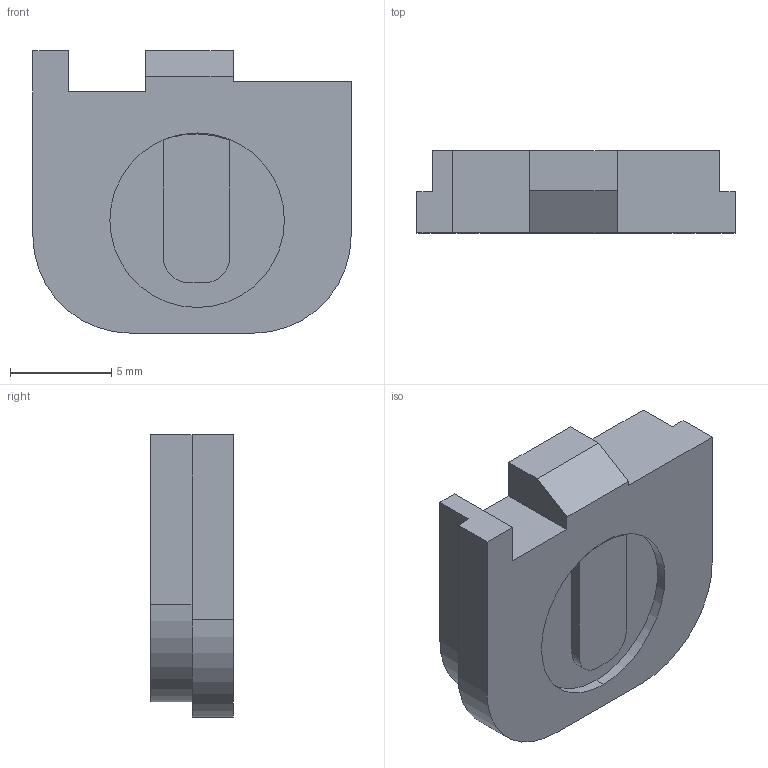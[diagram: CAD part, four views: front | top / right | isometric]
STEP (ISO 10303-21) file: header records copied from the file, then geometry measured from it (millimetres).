
FILE_DESCRIPTION (( 'STEP AP203' ), '1' );
FILE_NAME ('48BPv3.STEP', '2020-08-02T20:02:58', ( '' ), ( '' ), 'SwSTEP 2.0', 'SolidWorks 2020', '' );
FILE_SCHEMA (( 'CONFIG_CONTROL_DESIGN' ));
Length unit declared in the file: inch
Products named in the file (1): 48BPv3
Bounding box: 15.75 x 4.06 x 13.97 mm (x, y, z)
Volume: 699.2 mm3; surface area: 682.4 mm2
Topology: 2 solids, 2 shells, 32 faces, 81 edges, 54 vertices
Faces by surface type: plane 23, cylinder 8, bspline 1
Entity records: 1040 total; most frequent: CARTESIAN_POINT 177, ORIENTED_EDGE 162, DIRECTION 159, EDGE_CURVE 81, VECTOR 63, LINE 63, VERTEX_POINT 54, AXIS2_PLACEMENT_3D 48
